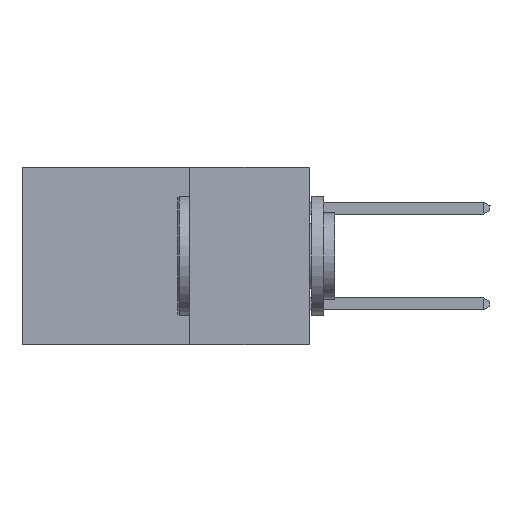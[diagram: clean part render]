
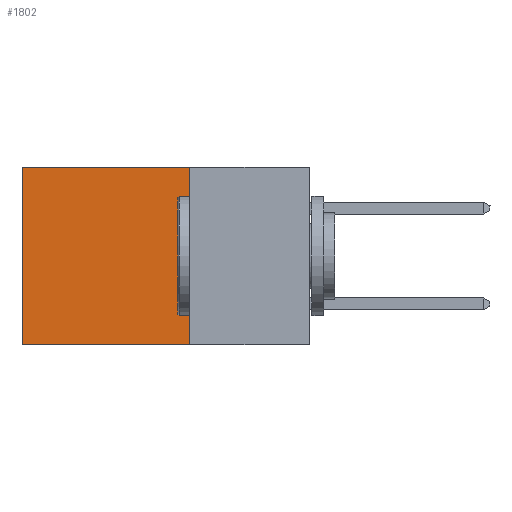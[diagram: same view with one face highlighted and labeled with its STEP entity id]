
A CAD part, left-side view. The second image highlights one B-rep face of the part: STEP entity #1802.
In plain terms, the highlighted planar face has unit normal (-1, 0, 0).
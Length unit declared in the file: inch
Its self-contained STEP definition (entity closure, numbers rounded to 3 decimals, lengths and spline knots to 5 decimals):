
#195 = CARTESIAN_POINT ( 'NONE',  ( 0.2875, 0.25, 0. ) ) ;
#1698 = EDGE_CURVE ( 'NONE', #15869, #8708, #5750, .T. ) ;
#1802 = ADVANCED_FACE ( 'NONE', ( #10777 ), #7700, .F. ) ;
#2309 = DIRECTION ( 'NONE',  ( 0., 0., -1. ) ) ;
#2339 = ORIENTED_EDGE ( 'NONE', *, *, #11111, .F. ) ;
#2527 = DIRECTION ( 'NONE',  ( 1., 0., 0. ) ) ;
#2684 = EDGE_CURVE ( 'NONE', #21281, #15869, #18198, .T. ) ;
#3812 = CARTESIAN_POINT ( 'NONE',  ( 0.2875, 0.25, 0. ) ) ;
#5329 = LINE ( 'NONE', #19948, #17815 ) ;
#5750 = LINE ( 'NONE', #19124, #9178 ) ;
#6298 = DIRECTION ( 'NONE',  ( 0., 1., 0. ) ) ;
#7620 = ORIENTED_EDGE ( 'NONE', *, *, #2684, .T. ) ;
#7700 = PLANE ( 'NONE',  #13277 ) ;
#7956 = CARTESIAN_POINT ( 'NONE',  ( 0.2875, 0.6, 0. ) ) ;
#8708 = VERTEX_POINT ( 'NONE', #13575 ) ;
#9178 = VECTOR ( 'NONE', #20807, 39.37008 ) ;
#9910 = DIRECTION ( 'NONE',  ( 0., 0., -1. ) ) ;
#10777 = FACE_OUTER_BOUND ( 'NONE', #16268, .T. ) ;
#11111 = EDGE_CURVE ( 'NONE', #21281, #21150, #5329, .T. ) ;
#11137 = ORIENTED_EDGE ( 'NONE', *, *, #1698, .T. ) ;
#11230 = ORIENTED_EDGE ( 'NONE', *, *, #12848, .F. ) ;
#11458 = CARTESIAN_POINT ( 'NONE',  ( 0.2875, 0.25, -0.37 ) ) ;
#12009 = CARTESIAN_POINT ( 'NONE',  ( 0.2875, 0.25, -0.37 ) ) ;
#12342 = VECTOR ( 'NONE', #16815, 39.37008 ) ;
#12848 = EDGE_CURVE ( 'NONE', #21150, #8708, #16671, .T. ) ;
#13277 = AXIS2_PLACEMENT_3D ( 'NONE', #21133, #2527, #2309 ) ;
#13575 = CARTESIAN_POINT ( 'NONE',  ( 0.2875, 0.6, -0.37 ) ) ;
#15869 = VERTEX_POINT ( 'NONE', #7956 ) ;
#16268 = EDGE_LOOP ( 'NONE', ( #11137, #11230, #2339, #7620 ) ) ;
#16671 = LINE ( 'NONE', #11458, #17983 ) ;
#16815 = DIRECTION ( 'NONE',  ( 0., 1., 0. ) ) ;
#17815 = VECTOR ( 'NONE', #9910, 39.37008 ) ;
#17983 = VECTOR ( 'NONE', #6298, 39.37008 ) ;
#18198 = LINE ( 'NONE', #195, #12342 ) ;
#19124 = CARTESIAN_POINT ( 'NONE',  ( 0.2875, 0.6, 0. ) ) ;
#19948 = CARTESIAN_POINT ( 'NONE',  ( 0.2875, 0.25, 0. ) ) ;
#20807 = DIRECTION ( 'NONE',  ( 0., 0., -1. ) ) ;
#21133 = CARTESIAN_POINT ( 'NONE',  ( 0.2875, 0.25, 0. ) ) ;
#21150 = VERTEX_POINT ( 'NONE', #12009 ) ;
#21281 = VERTEX_POINT ( 'NONE', #3812 ) ;
